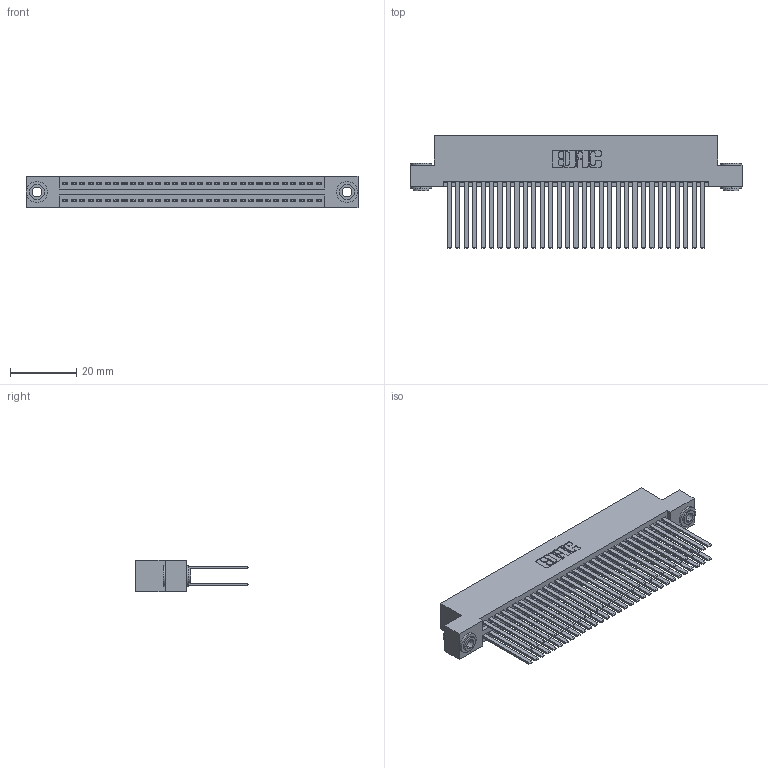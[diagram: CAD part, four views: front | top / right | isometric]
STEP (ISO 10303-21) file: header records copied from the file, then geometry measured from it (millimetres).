
FILE_DESCRIPTION (( 'STEP AP203' ), '1' );
FILE_NAME ('345-062-544-203.STEP', '2018-09-27T15:54:00', ( '' ), ( '' ), 'SwSTEP 2.0', 'SolidWorks 2016', '' );
FILE_SCHEMA (( 'CONFIG_CONTROL_DESIGN' ));
Length unit declared in the file: inch
Products named in the file (4): 345-292-001_345-293-144; 345-250-002_345-250-002-102; 345-062-544-203; 345 Part_Flush Mounting Lugs - 0.156 Dia-TH
Assembly tree (65 placements, depth 2):
  345-062-544-203
    345 Part_Flush Mounting Lugs - 0.156 Dia-TH
    345-292-001_345-293-144  x62
    345-250-002_345-250-002-102  x2
Bounding box: 99.95 x 33.96 x 9.4 mm (x, y, z)
Volume: 10495.6 mm3; surface area: 18053.4 mm2
Topology: 65 solids, 65 shells, 2892 faces, 8539 edges, 5606 vertices
Faces by surface type: plane 1888, cylinder 996, cone 8
Entity records: 26270 total; most frequent: CARTESIAN_POINT 4387, ORIENTED_EDGE 4314, DIRECTION 3911, EDGE_CURVE 2157, VECTOR 1881, LINE 1881, VERTEX_POINT 1434, AXIS2_PLACEMENT_3D 1015
